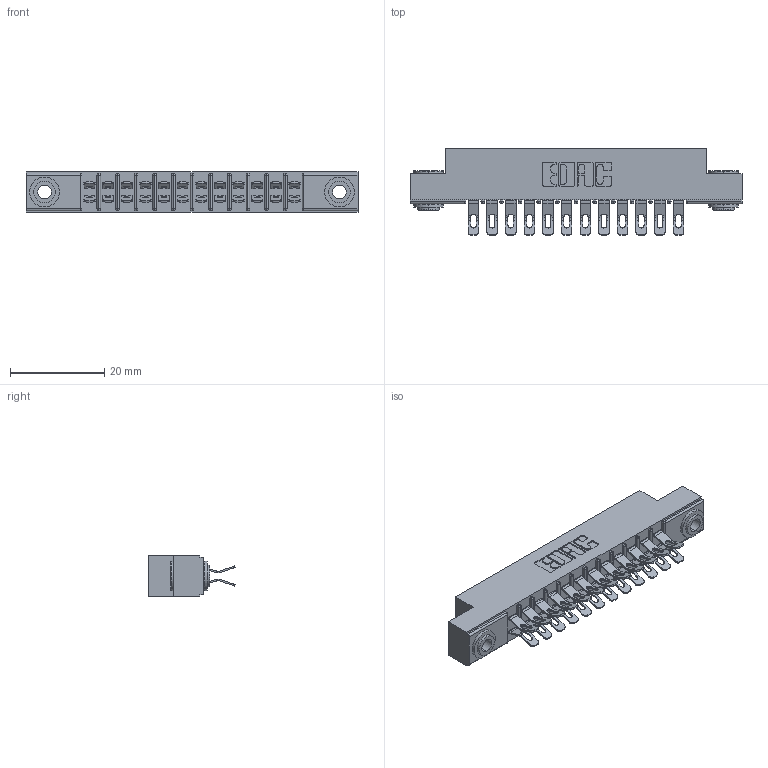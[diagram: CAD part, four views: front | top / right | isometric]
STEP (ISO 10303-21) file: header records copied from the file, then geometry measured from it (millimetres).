
FILE_DESCRIPTION (( 'STEP AP203' ), '1' );
FILE_NAME ('355-024-555-203.STEP', '2019-09-11T04:56:39', ( '' ), ( '' ), 'SwSTEP 2.0', 'SolidWorks 2016', '' );
FILE_SCHEMA (( 'CONFIG_CONTROL_DESIGN' ));
Length unit declared in the file: inch
Products named in the file (4): 355-024-555-203; 305 Part_.156 Dia; 305-290-001_555; 345-250-002_345-250-002-102
Assembly tree (27 placements, depth 2):
  355-024-555-203
    305 Part_.156 Dia
    305-290-001_555  x24
    345-250-002_345-250-002-102  x2
Bounding box: 70.56 x 18.41 x 8.71 mm (x, y, z)
Volume: 4508.8 mm3; surface area: 8591.4 mm2
Topology: 27 solids, 27 shells, 1752 faces, 5168 edges, 3376 vertices
Faces by surface type: plane 860, cylinder 836, sphere 48, cone 8
Entity records: 18334 total; most frequent: CARTESIAN_POINT 3033, ORIENTED_EDGE 2988, DIRECTION 2968, EDGE_CURVE 1494, VECTOR 1146, LINE 1146, VERTEX_POINT 960, AXIS2_PLACEMENT_3D 911
